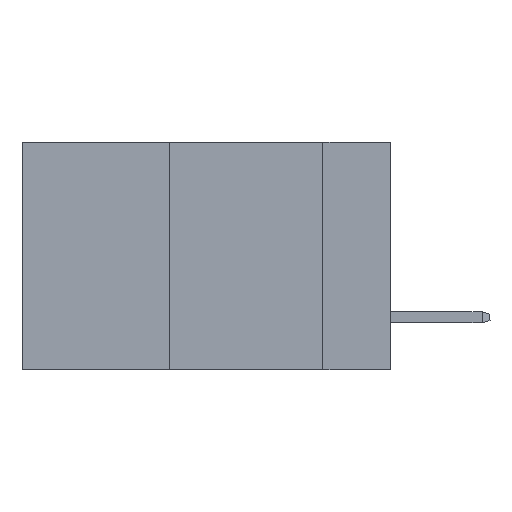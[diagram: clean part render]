
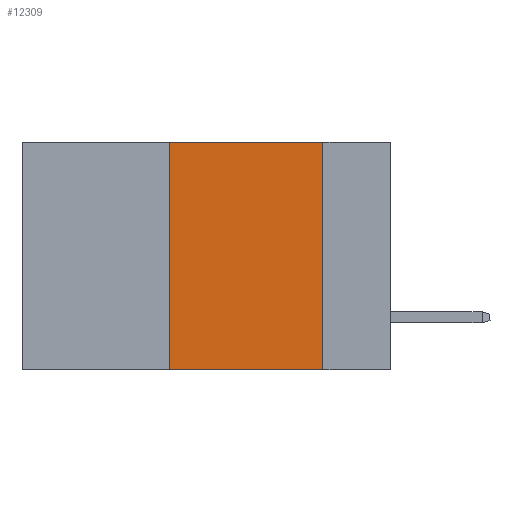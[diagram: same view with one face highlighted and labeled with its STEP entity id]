
A CAD part, left-side view. The second image highlights one B-rep face of the part: STEP entity #12309.
In plain terms, the highlighted planar face has unit normal (-1, 0, 0).
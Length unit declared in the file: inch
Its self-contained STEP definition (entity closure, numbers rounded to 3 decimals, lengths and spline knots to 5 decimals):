
#312 = ORIENTED_EDGE ( 'NONE', *, *, #12467, .F. ) ;
#1708 = ORIENTED_EDGE ( 'NONE', *, *, #9859, .F. ) ;
#2171 = EDGE_CURVE ( 'NONE', #10576, #4812, #11832, .T. ) ;
#2229 = DIRECTION ( 'NONE',  ( 1., 0., 0. ) ) ;
#4812 = VERTEX_POINT ( 'NONE', #7014 ) ;
#5173 = EDGE_CURVE ( 'NONE', #7471, #4812, #11765, .T. ) ;
#5675 = PLANE ( 'NONE',  #12204 ) ;
#5727 = DIRECTION ( 'NONE',  ( 0., 0., 1. ) ) ;
#6371 = VERTEX_POINT ( 'NONE', #13985 ) ;
#6511 = DIRECTION ( 'NONE',  ( 0., 0., -1. ) ) ;
#6926 = ORIENTED_EDGE ( 'NONE', *, *, #2171, .T. ) ;
#7014 = CARTESIAN_POINT ( 'NONE',  ( 0., 0.11, -0.37 ) ) ;
#7471 = VERTEX_POINT ( 'NONE', #10249 ) ;
#7817 = VECTOR ( 'NONE', #5727, 39.37008 ) ;
#7963 = ORIENTED_EDGE ( 'NONE', *, *, #5173, .F. ) ;
#8284 = FACE_OUTER_BOUND ( 'NONE', #13365, .T. ) ;
#8801 = VECTOR ( 'NONE', #11557, 39.37008 ) ;
#8882 = CARTESIAN_POINT ( 'NONE',  ( 0., 0.6, -0.37 ) ) ;
#8930 = DIRECTION ( 'NONE',  ( 0., -1., 0. ) ) ;
#9070 = CARTESIAN_POINT ( 'NONE',  ( 0., 0.6, 0. ) ) ;
#9110 = CARTESIAN_POINT ( 'NONE',  ( 0., 0.36, -0.37 ) ) ;
#9859 = EDGE_CURVE ( 'NONE', #10576, #6371, #13323, .T. ) ;
#10174 = DIRECTION ( 'NONE',  ( 0., 0., -1. ) ) ;
#10249 = CARTESIAN_POINT ( 'NONE',  ( 0., 0.11, 0. ) ) ;
#10462 = CARTESIAN_POINT ( 'NONE',  ( 0., 0.6, 0. ) ) ;
#10576 = VERTEX_POINT ( 'NONE', #9110 ) ;
#11439 = VECTOR ( 'NONE', #6511, 39.37008 ) ;
#11496 = VECTOR ( 'NONE', #8930, 39.37008 ) ;
#11557 = DIRECTION ( 'NONE',  ( 0., -1., 0. ) ) ;
#11717 = LINE ( 'NONE', #10462, #8801 ) ;
#11765 = LINE ( 'NONE', #14156, #11439 ) ;
#11832 = LINE ( 'NONE', #8882, #11496 ) ;
#12204 = AXIS2_PLACEMENT_3D ( 'NONE', #9070, #2229, #10174 ) ;
#12309 = ADVANCED_FACE ( 'NONE', ( #8284 ), #5675, .F. ) ;
#12367 = CARTESIAN_POINT ( 'NONE',  ( 0., 0.36, 0. ) ) ;
#12467 = EDGE_CURVE ( 'NONE', #6371, #7471, #11717, .T. ) ;
#13323 = LINE ( 'NONE', #12367, #7817 ) ;
#13365 = EDGE_LOOP ( 'NONE', ( #7963, #312, #1708, #6926 ) ) ;
#13985 = CARTESIAN_POINT ( 'NONE',  ( 0., 0.36, 0. ) ) ;
#14156 = CARTESIAN_POINT ( 'NONE',  ( 0., 0.11, 0. ) ) ;
